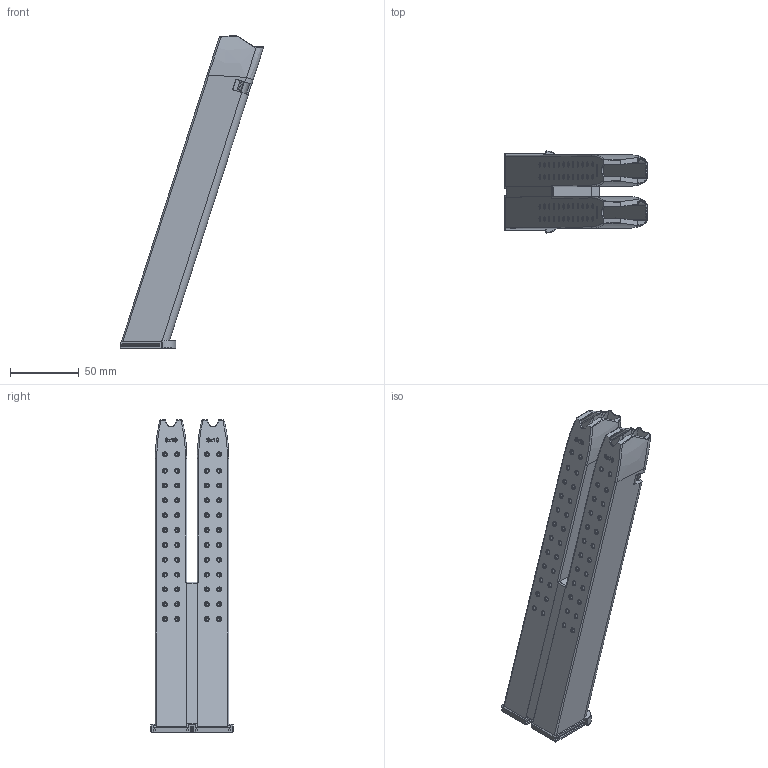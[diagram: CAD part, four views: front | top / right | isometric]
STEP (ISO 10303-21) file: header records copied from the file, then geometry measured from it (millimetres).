
FILE_DESCRIPTION(/* description */ (''),/* implementation_level */ '2;1');
FILE_NAME(/* name */ 'Glocknofsky Big Stick v1.step',/* time_stamp */ '2022-03-26T10:53:36-04:00',/* author */ (''),/* organization */ (''),/* preprocessor_version */ 'ST-DEVELOPER v18.1',/* originating_system */ 'Autodesk Translation Framework v10.13.0.1454',/* authorisation */ '');
FILE_SCHEMA (('AUTOMOTIVE_DESIGN { 1 0 10303 214 3 1 1 }'));
Products named in the file (2): Glocknofsky Big Stick; glocknofsky mag body
Assembly tree (1 placements, depth 2):
  Glocknofsky Big Stick
    glocknofsky mag body
Bounding box: 104.45 x 59.73 x 227.9 mm (x, y, z)
Volume: 121839.6 mm3; surface area: 92201.6 mm2
Topology: 1 solids, 51 shells, 2200 faces, 5977 edges, 3903 vertices
Faces by surface type: bspline 1224, plane 727, cylinder 137, torus 96, sphere 16
Entity records: 93522 total; most frequent: CARTESIAN_POINT 45975, ORIENTED_EDGE 11950, DIRECTION 6034, EDGE_CURVE 5975, VERTEX_POINT 3903, LINE 2822, VECTOR 2822, B_SPLINE_CURVE_WITH_KNOTS 2524
